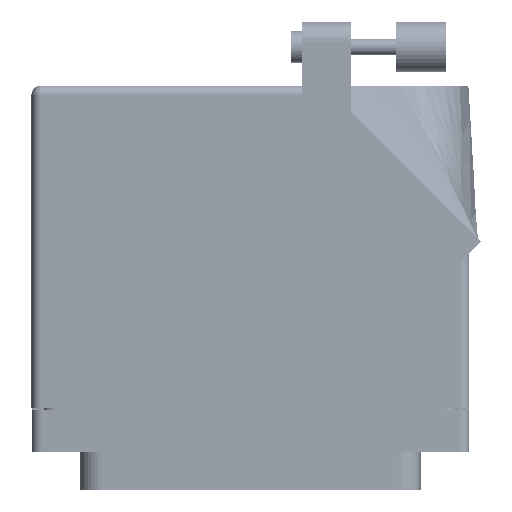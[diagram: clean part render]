
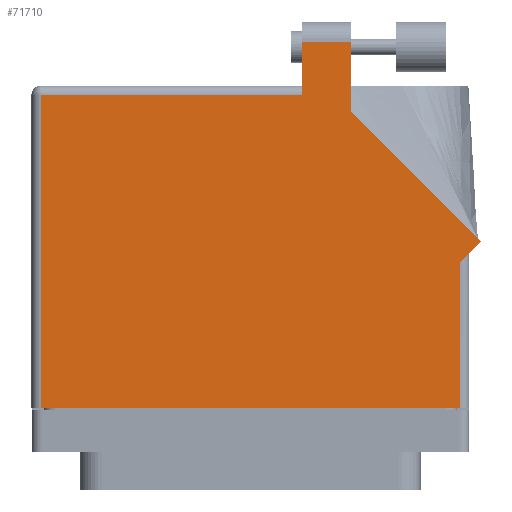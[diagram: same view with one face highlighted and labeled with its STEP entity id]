
A CAD part, front view. The second image highlights one B-rep face of the part: STEP entity #71710.
In plain terms, the highlighted face is planar.
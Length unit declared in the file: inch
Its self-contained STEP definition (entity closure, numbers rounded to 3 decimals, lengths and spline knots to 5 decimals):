
#956 = EDGE_LOOP ( 'NONE', ( #6955, #85190, #23893, #90293, #63603, #79946, #86649, #80870, #41366 ) ) ;
#2995 = VERTEX_POINT ( 'NONE', #87569 ) ;
#3260 = DIRECTION ( 'NONE',  ( 0., -1., 0. ) ) ;
#4355 = CARTESIAN_POINT ( 'NONE',  ( 0.6345, 2.205, 0.765 ) ) ;
#5877 = PLANE ( 'NONE',  #44667 ) ;
#6955 = ORIENTED_EDGE ( 'NONE', *, *, #66194, .T. ) ;
#8091 = EDGE_CURVE ( 'NONE', #44141, #2995, #35624, .T. ) ;
#9772 = CARTESIAN_POINT ( 'NONE',  ( -1.3775, 1.868, 0.765 ) ) ;
#13494 = CARTESIAN_POINT ( 'NONE',  ( -1.3155, -0.1, 0.765 ) ) ;
#14131 = VECTOR ( 'NONE', #19206, 39.37008 ) ;
#17988 = VERTEX_POINT ( 'NONE', #78952 ) ;
#18977 = VERTEX_POINT ( 'NONE', #4355 ) ;
#19206 = DIRECTION ( 'NONE',  ( 0., 1., 0. ) ) ;
#19979 = DIRECTION ( 'NONE',  ( -1., 0., 0. ) ) ;
#22462 = VERTEX_POINT ( 'NONE', #13494 ) ;
#22767 = VECTOR ( 'NONE', #27678, 39.37008 ) ;
#23893 = ORIENTED_EDGE ( 'NONE', *, *, #66209, .T. ) ;
#24569 = CARTESIAN_POINT ( 'NONE',  ( 1.44821, 0.95071, 0.765 ) ) ;
#25400 = LINE ( 'NONE', #44673, #79910 ) ;
#26322 = EDGE_CURVE ( 'NONE', #46309, #54477, #52556, .T. ) ;
#27415 = EDGE_CURVE ( 'NONE', #76672, #17988, #60335, .T. ) ;
#27678 = DIRECTION ( 'NONE',  ( 0., 1., 0. ) ) ;
#27686 = EDGE_CURVE ( 'NONE', #22462, #44141, #30103, .T. ) ;
#30103 = LINE ( 'NONE', #51267, #47656 ) ;
#30292 = DIRECTION ( 'NONE',  ( -1., 0., 0. ) ) ;
#30842 = VECTOR ( 'NONE', #88126, 39.37008 ) ;
#31901 = LINE ( 'NONE', #69079, #14131 ) ;
#32979 = VECTOR ( 'NONE', #30292, 39.37008 ) ;
#35120 = EDGE_CURVE ( 'NONE', #54477, #22462, #25400, .T. ) ;
#35265 = VERTEX_POINT ( 'NONE', #58276 ) ;
#35624 = LINE ( 'NONE', #57762, #22767 ) ;
#38097 = VECTOR ( 'NONE', #3260, 39.37008 ) ;
#41366 = ORIENTED_EDGE ( 'NONE', *, *, #27415, .T. ) ;
#44141 = VERTEX_POINT ( 'NONE', #87053 ) ;
#44667 = AXIS2_PLACEMENT_3D ( 'NONE', #48631, #85327, #19979 ) ;
#44673 = CARTESIAN_POINT ( 'NONE',  ( -1.3155, -0.1, 0.765 ) ) ;
#46061 = DIRECTION ( 'NONE',  ( 0., -1., 0. ) ) ;
#46309 = VERTEX_POINT ( 'NONE', #85002 ) ;
#47185 = VECTOR ( 'NONE', #60111, 39.37008 ) ;
#47656 = VECTOR ( 'NONE', #79989, 39.37008 ) ;
#48631 = CARTESIAN_POINT ( 'NONE',  ( -1.3775, 1.93, 0.765 ) ) ;
#49724 = LINE ( 'NONE', #87669, #32979 ) ;
#51267 = CARTESIAN_POINT ( 'NONE',  ( -1.3775, -0.1, 0.765 ) ) ;
#52403 = LINE ( 'NONE', #82002, #30842 ) ;
#52556 = LINE ( 'NONE', #9772, #47185 ) ;
#53203 = EDGE_CURVE ( 'NONE', #2995, #76672, #52403, .T. ) ;
#54477 = VERTEX_POINT ( 'NONE', #74064 ) ;
#57762 = CARTESIAN_POINT ( 'NONE',  ( 1.3155, 0.88, 0.765 ) ) ;
#58276 = CARTESIAN_POINT ( 'NONE',  ( 0.3275, 2.205, 0.765 ) ) ;
#60111 = DIRECTION ( 'NONE',  ( -1., 0., 0. ) ) ;
#60335 = LINE ( 'NONE', #24569, #65425 ) ;
#63603 = ORIENTED_EDGE ( 'NONE', *, *, #35120, .T. ) ;
#65425 = VECTOR ( 'NONE', #76275, 39.37008 ) ;
#66194 = EDGE_CURVE ( 'NONE', #17988, #18977, #31901, .T. ) ;
#66209 = EDGE_CURVE ( 'NONE', #35265, #46309, #75207, .T. ) ;
#69079 = CARTESIAN_POINT ( 'NONE',  ( 0.6345, 1.76442, 0.765 ) ) ;
#71663 = CARTESIAN_POINT ( 'NONE',  ( 1.44821, 0.95071, 0.765 ) ) ;
#71686 = FACE_OUTER_BOUND ( 'NONE', #956, .T. ) ;
#71710 = ADVANCED_FACE ( 'NONE', ( #71686 ), #5877, .F. ) ;
#74064 = CARTESIAN_POINT ( 'NONE',  ( -1.3155, 1.868, 0.765 ) ) ;
#74348 = EDGE_CURVE ( 'NONE', #18977, #35265, #49724, .T. ) ;
#75207 = LINE ( 'NONE', #90655, #38097 ) ;
#76275 = DIRECTION ( 'NONE',  ( -0.707, 0.707, 0. ) ) ;
#76672 = VERTEX_POINT ( 'NONE', #71663 ) ;
#78952 = CARTESIAN_POINT ( 'NONE',  ( 0.6345, 1.76442, 0.765 ) ) ;
#79910 = VECTOR ( 'NONE', #46061, 39.37008 ) ;
#79946 = ORIENTED_EDGE ( 'NONE', *, *, #27686, .T. ) ;
#79989 = DIRECTION ( 'NONE',  ( 1., 0., 0. ) ) ;
#80870 = ORIENTED_EDGE ( 'NONE', *, *, #53203, .T. ) ;
#82002 = CARTESIAN_POINT ( 'NONE',  ( 1.3775, 0.88, 0.765 ) ) ;
#85002 = CARTESIAN_POINT ( 'NONE',  ( 0.3275, 1.868, 0.765 ) ) ;
#85190 = ORIENTED_EDGE ( 'NONE', *, *, #74348, .T. ) ;
#85327 = DIRECTION ( 'NONE',  ( 0., 0., -1. ) ) ;
#86649 = ORIENTED_EDGE ( 'NONE', *, *, #8091, .T. ) ;
#87053 = CARTESIAN_POINT ( 'NONE',  ( 1.3155, -0.1, 0.765 ) ) ;
#87569 = CARTESIAN_POINT ( 'NONE',  ( 1.3155, 0.818, 0.765 ) ) ;
#87669 = CARTESIAN_POINT ( 'NONE',  ( 0.3275, 2.205, 0.765 ) ) ;
#88126 = DIRECTION ( 'NONE',  ( 0.707, 0.707, 0. ) ) ;
#90293 = ORIENTED_EDGE ( 'NONE', *, *, #26322, .T. ) ;
#90655 = CARTESIAN_POINT ( 'NONE',  ( 0.3275, 1.93, 0.765 ) ) ;
